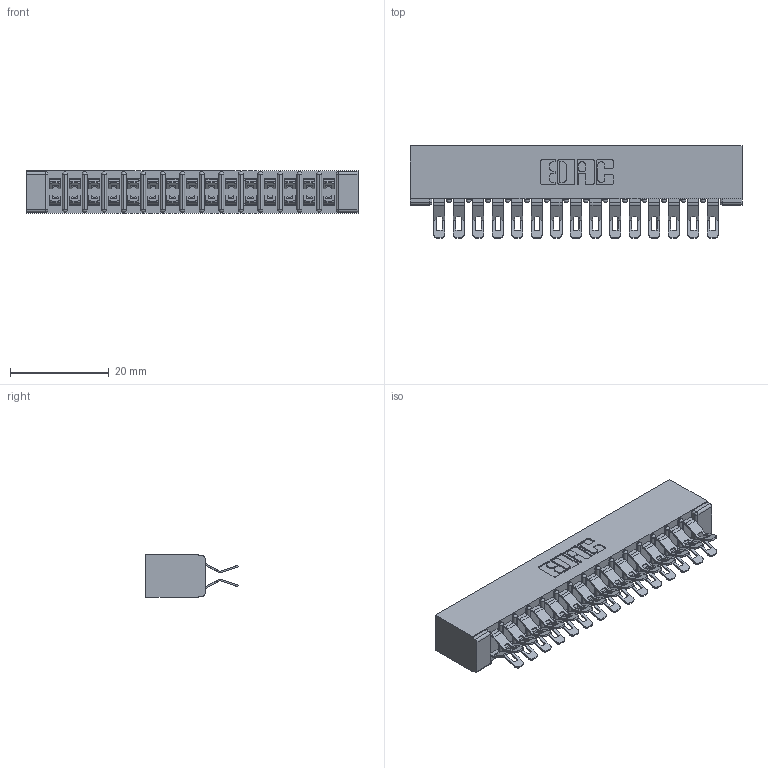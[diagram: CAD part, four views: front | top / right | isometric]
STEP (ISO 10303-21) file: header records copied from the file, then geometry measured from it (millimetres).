
FILE_DESCRIPTION (( 'STEP AP203' ), '1' );
FILE_NAME ('357-030-455-201.STEP', '2020-10-03T13:27:17', ( '' ), ( '' ), 'SwSTEP 2.0', 'SolidWorks 2020', '' );
FILE_SCHEMA (( 'CONFIG_CONTROL_DESIGN' ));
Length unit declared in the file: inch
Products named in the file (3): 307-290-001_555; 307 Part_No Mounting Lugs; 357-030-455-201
Assembly tree (31 placements, depth 2):
  357-030-455-201
    307 Part_No Mounting Lugs
    307-290-001_555  x30
Bounding box: 67.31 x 18.75 x 8.71 mm (x, y, z)
Volume: 4726.1 mm3; surface area: 8946.7 mm2
Topology: 31 solids, 31 shells, 1956 faces, 5729 edges, 3734 vertices
Faces by surface type: plane 1086, cylinder 838, sphere 32
Entity records: 16927 total; most frequent: CARTESIAN_POINT 2779, ORIENTED_EDGE 2752, DIRECTION 2740, EDGE_CURVE 1376, LINE 1034, VECTOR 1034, VERTEX_POINT 892, AXIS2_PLACEMENT_3D 853
